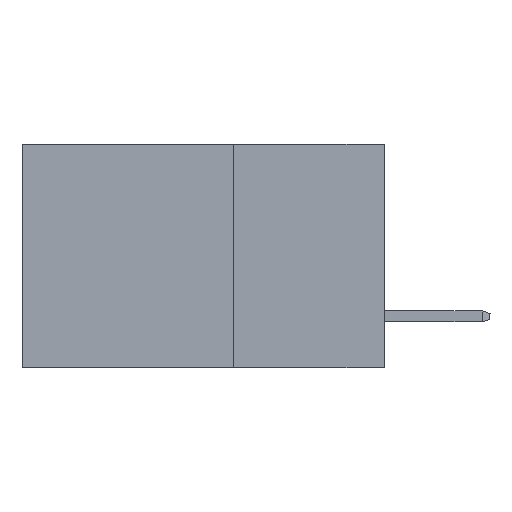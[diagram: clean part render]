
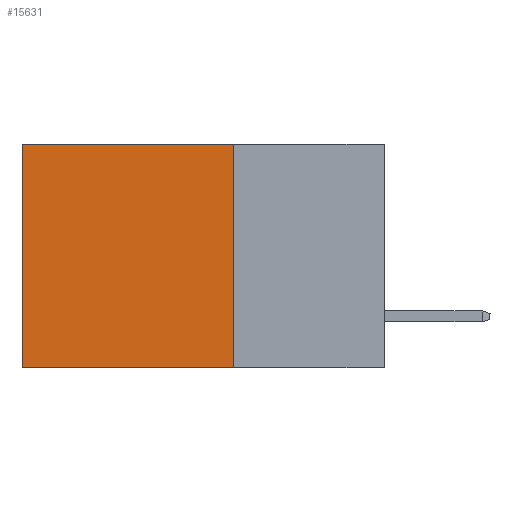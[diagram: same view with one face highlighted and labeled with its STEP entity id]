
A CAD part, left-side view. The second image highlights one B-rep face of the part: STEP entity #15631.
In plain terms, the highlighted planar face has unit normal (-1, 0, 0).
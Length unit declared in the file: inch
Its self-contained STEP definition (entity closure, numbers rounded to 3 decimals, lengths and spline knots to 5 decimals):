
#21 = EDGE_LOOP ( 'NONE', ( #5785, #18735, #22460, #16152 ) ) ;
#160 = VECTOR ( 'NONE', #15839, 39.37008 ) ;
#1818 = FACE_OUTER_BOUND ( 'NONE', #21, .T. ) ;
#2352 = EDGE_CURVE ( 'NONE', #14320, #19338, #9368, .T. ) ;
#2375 = DIRECTION ( 'NONE',  ( 0., 0., -1. ) ) ;
#2526 = LINE ( 'NONE', #23550, #160 ) ;
#2555 = DIRECTION ( 'NONE',  ( 0., 0., -1. ) ) ;
#3552 = VECTOR ( 'NONE', #9618, 39.37008 ) ;
#3769 = CARTESIAN_POINT ( 'NONE',  ( 0.2615, 0.25, 0. ) ) ;
#4068 = EDGE_CURVE ( 'NONE', #19338, #22427, #2526, .T. ) ;
#5785 = ORIENTED_EDGE ( 'NONE', *, *, #5996, .T. ) ;
#5996 = EDGE_CURVE ( 'NONE', #21737, #22427, #15438, .T. ) ;
#7269 = DIRECTION ( 'NONE',  ( 1., 0., 0. ) ) ;
#7523 = PLANE ( 'NONE',  #12954 ) ;
#7724 = VECTOR ( 'NONE', #2375, 39.37008 ) ;
#9368 = LINE ( 'NONE', #11332, #3552 ) ;
#9618 = DIRECTION ( 'NONE',  ( 0., 0., -1. ) ) ;
#11332 = CARTESIAN_POINT ( 'NONE',  ( 0.2615, 0.25, -0.37 ) ) ;
#11887 = CARTESIAN_POINT ( 'NONE',  ( 0.2615, 0.6, -0.37 ) ) ;
#12869 = VECTOR ( 'NONE', #15232, 39.37008 ) ;
#12954 = AXIS2_PLACEMENT_3D ( 'NONE', #24090, #7269, #2555 ) ;
#13131 = CARTESIAN_POINT ( 'NONE',  ( 0.2615, 0.6, -0.37 ) ) ;
#14320 = VERTEX_POINT ( 'NONE', #23326 ) ;
#15232 = DIRECTION ( 'NONE',  ( 0., 1., 0. ) ) ;
#15438 = LINE ( 'NONE', #11887, #7724 ) ;
#15631 = ADVANCED_FACE ( 'NONE', ( #1818 ), #7523, .F. ) ;
#15839 = DIRECTION ( 'NONE',  ( 0., 1., 0. ) ) ;
#16152 = ORIENTED_EDGE ( 'NONE', *, *, #17257, .T. ) ;
#16823 = LINE ( 'NONE', #3769, #12869 ) ;
#17257 = EDGE_CURVE ( 'NONE', #14320, #21737, #16823, .T. ) ;
#17345 = CARTESIAN_POINT ( 'NONE',  ( 0.2615, 0.6, 0. ) ) ;
#18391 = CARTESIAN_POINT ( 'NONE',  ( 0.2615, 0.25, -0.37 ) ) ;
#18735 = ORIENTED_EDGE ( 'NONE', *, *, #4068, .F. ) ;
#19338 = VERTEX_POINT ( 'NONE', #18391 ) ;
#21737 = VERTEX_POINT ( 'NONE', #17345 ) ;
#22427 = VERTEX_POINT ( 'NONE', #13131 ) ;
#22460 = ORIENTED_EDGE ( 'NONE', *, *, #2352, .F. ) ;
#23326 = CARTESIAN_POINT ( 'NONE',  ( 0.2615, 0.25, 0. ) ) ;
#23550 = CARTESIAN_POINT ( 'NONE',  ( 0.2615, 0.25, -0.37 ) ) ;
#24090 = CARTESIAN_POINT ( 'NONE',  ( 0.2615, 0.25, -0.37 ) ) ;
